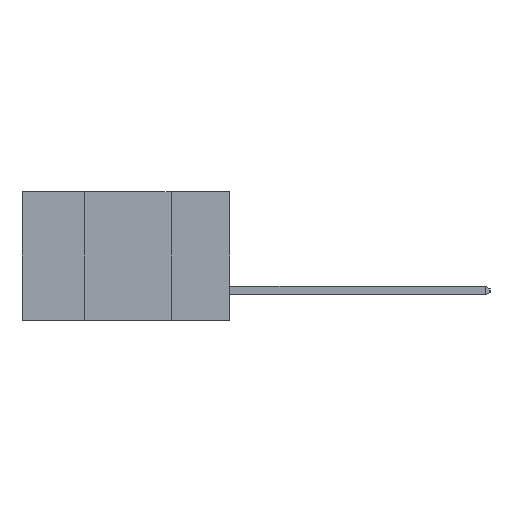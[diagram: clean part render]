
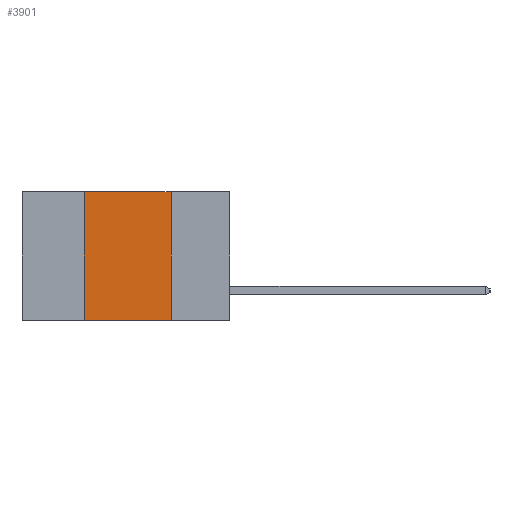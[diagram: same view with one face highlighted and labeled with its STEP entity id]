
A CAD part, left-side view. The second image highlights one B-rep face of the part: STEP entity #3901.
In plain terms, the highlighted planar face has unit normal (-1, 0, 0).
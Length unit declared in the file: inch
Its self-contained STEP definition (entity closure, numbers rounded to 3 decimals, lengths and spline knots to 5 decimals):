
#795 = VERTEX_POINT ( 'NONE', #3004 ) ;
#948 = CARTESIAN_POINT ( 'NONE',  ( 0., 0.6, 0. ) ) ;
#1075 = CARTESIAN_POINT ( 'NONE',  ( 0., 0.42, 0. ) ) ;
#2064 = VECTOR ( 'NONE', #3810, 39.37008 ) ;
#2162 = DIRECTION ( 'NONE',  ( 0., -1., 0. ) ) ;
#2300 = DIRECTION ( 'NONE',  ( 0., 0., -1. ) ) ;
#3004 = CARTESIAN_POINT ( 'NONE',  ( 0., 0.17, -0.37 ) ) ;
#3281 = EDGE_LOOP ( 'NONE', ( #15064, #17266, #11242, #17922 ) ) ;
#3810 = DIRECTION ( 'NONE',  ( 0., 0., 1. ) ) ;
#3833 = DIRECTION ( 'NONE',  ( 0., 0., -1. ) ) ;
#3852 = DIRECTION ( 'NONE',  ( 1., 0., 0. ) ) ;
#3901 = ADVANCED_FACE ( 'NONE', ( #6094 ), #7752, .F. ) ;
#4030 = EDGE_CURVE ( 'NONE', #7517, #795, #14960, .T. ) ;
#4358 = CARTESIAN_POINT ( 'NONE',  ( 0., 0.17, 0. ) ) ;
#5253 = AXIS2_PLACEMENT_3D ( 'NONE', #7204, #3852, #3833 ) ;
#5405 = VECTOR ( 'NONE', #2162, 39.37008 ) ;
#6094 = FACE_OUTER_BOUND ( 'NONE', #3281, .T. ) ;
#7204 = CARTESIAN_POINT ( 'NONE',  ( 0., 0.6, 0. ) ) ;
#7251 = VECTOR ( 'NONE', #2300, 39.37008 ) ;
#7517 = VERTEX_POINT ( 'NONE', #14388 ) ;
#7752 = PLANE ( 'NONE',  #5253 ) ;
#7821 = EDGE_CURVE ( 'NONE', #10018, #795, #10222, .T. ) ;
#8329 = CARTESIAN_POINT ( 'NONE',  ( 0., 0.42, -0.37 ) ) ;
#8950 = LINE ( 'NONE', #948, #9387 ) ;
#9387 = VECTOR ( 'NONE', #16913, 39.37008 ) ;
#10018 = VERTEX_POINT ( 'NONE', #8329 ) ;
#10222 = LINE ( 'NONE', #13885, #5405 ) ;
#11242 = ORIENTED_EDGE ( 'NONE', *, *, #15392, .F. ) ;
#12550 = CARTESIAN_POINT ( 'NONE',  ( 0., 0.42, 0. ) ) ;
#13885 = CARTESIAN_POINT ( 'NONE',  ( 0., 0.6, -0.37 ) ) ;
#14388 = CARTESIAN_POINT ( 'NONE',  ( 0., 0.17, 0. ) ) ;
#14960 = LINE ( 'NONE', #4358, #7251 ) ;
#15064 = ORIENTED_EDGE ( 'NONE', *, *, #4030, .F. ) ;
#15392 = EDGE_CURVE ( 'NONE', #10018, #16155, #16627, .T. ) ;
#16155 = VERTEX_POINT ( 'NONE', #1075 ) ;
#16627 = LINE ( 'NONE', #12550, #2064 ) ;
#16913 = DIRECTION ( 'NONE',  ( 0., -1., 0. ) ) ;
#17266 = ORIENTED_EDGE ( 'NONE', *, *, #18112, .F. ) ;
#17922 = ORIENTED_EDGE ( 'NONE', *, *, #7821, .T. ) ;
#18112 = EDGE_CURVE ( 'NONE', #16155, #7517, #8950, .T. ) ;
